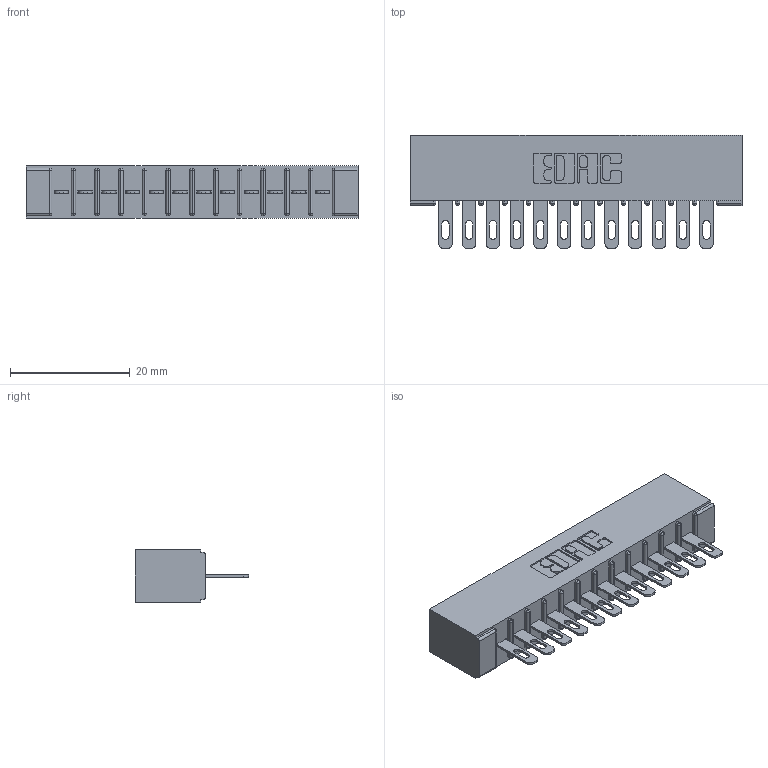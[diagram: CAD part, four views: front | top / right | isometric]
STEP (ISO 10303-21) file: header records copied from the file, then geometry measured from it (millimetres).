
FILE_DESCRIPTION (( 'STEP AP203' ), '1' );
FILE_NAME ('316-012-500-101.STEP', '2018-07-31T00:21:05', ( '' ), ( '' ), 'SwSTEP 2.0', 'SolidWorks 2016', '' );
FILE_SCHEMA (( 'CONFIG_CONTROL_DESIGN' ));
Length unit declared in the file: inch
Products named in the file (3): 306-290-001_100; 316-012-500-101; 306 Part_No Mounting
Assembly tree (13 placements, depth 2):
  316-012-500-101
    306 Part_No Mounting
    306-290-001_100  x12
Bounding box: 55.42 x 18.87 x 8.71 mm (x, y, z)
Volume: 4065.6 mm3; surface area: 6136.1 mm2
Topology: 13 solids, 13 shells, 1020 faces, 2872 edges, 1848 vertices
Faces by surface type: plane 664, cylinder 308, sphere 48
Entity records: 14963 total; most frequent: CARTESIAN_POINT 2507, ORIENTED_EDGE 2480, DIRECTION 2476, EDGE_CURVE 1240, LINE 954, VECTOR 954, VERTEX_POINT 792, AXIS2_PLACEMENT_3D 761
